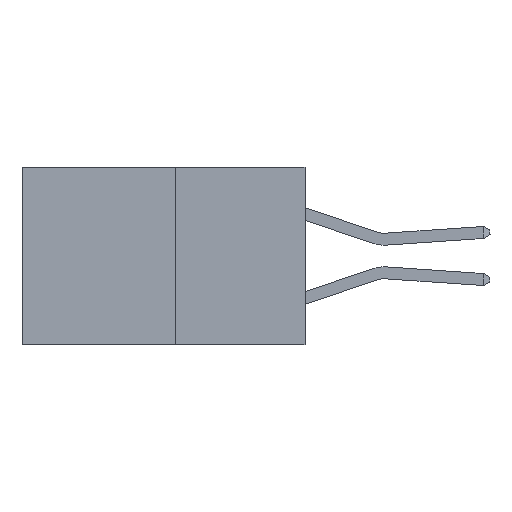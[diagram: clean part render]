
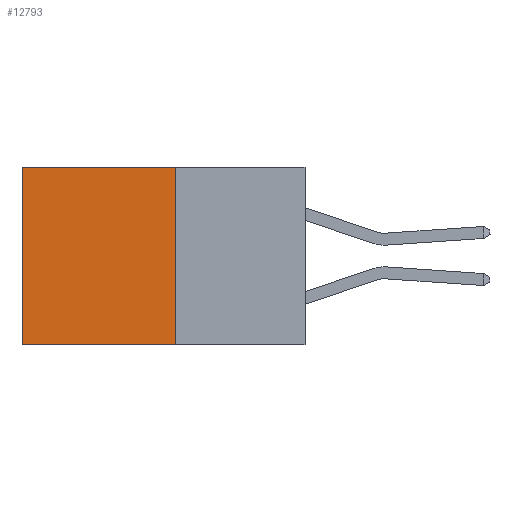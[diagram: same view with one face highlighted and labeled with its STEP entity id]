
A CAD part, left-side view. The second image highlights one B-rep face of the part: STEP entity #12793.
In plain terms, the highlighted planar face has unit normal (-1, 0, 0).
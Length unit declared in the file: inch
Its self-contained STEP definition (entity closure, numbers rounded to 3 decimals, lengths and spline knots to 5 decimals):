
#480 = PLANE ( 'NONE',  #8876 ) ;
#531 = VECTOR ( 'NONE', #13611, 39.37008 ) ;
#1140 = LINE ( 'NONE', #5750, #3578 ) ;
#1280 = EDGE_CURVE ( 'NONE', #2827, #8145, #3301, .T. ) ;
#2827 = VERTEX_POINT ( 'NONE', #12738 ) ;
#2942 = EDGE_LOOP ( 'NONE', ( #7919, #4447, #13223, #12456 ) ) ;
#3301 = LINE ( 'NONE', #7163, #531 ) ;
#3568 = VECTOR ( 'NONE', #4720, 39.37008 ) ;
#3578 = VECTOR ( 'NONE', #6773, 39.37008 ) ;
#3621 = CARTESIAN_POINT ( 'NONE',  ( 0.277, 0.27, -0.37 ) ) ;
#3948 = DIRECTION ( 'NONE',  ( 0., 1., 0. ) ) ;
#4089 = CARTESIAN_POINT ( 'NONE',  ( 0.277, 0.27, -0.37 ) ) ;
#4447 = ORIENTED_EDGE ( 'NONE', *, *, #6210, .F. ) ;
#4533 = CARTESIAN_POINT ( 'NONE',  ( 0.277, 0.27, 0. ) ) ;
#4691 = DIRECTION ( 'NONE',  ( 1., 0., 0. ) ) ;
#4720 = DIRECTION ( 'NONE',  ( 0., 1., 0. ) ) ;
#5750 = CARTESIAN_POINT ( 'NONE',  ( 0.277, 0.27, -0.37 ) ) ;
#6001 = EDGE_CURVE ( 'NONE', #9197, #6017, #1140, .T. ) ;
#6017 = VERTEX_POINT ( 'NONE', #7365 ) ;
#6210 = EDGE_CURVE ( 'NONE', #6017, #8145, #12204, .T. ) ;
#6541 = EDGE_CURVE ( 'NONE', #9197, #2827, #8198, .T. ) ;
#6773 = DIRECTION ( 'NONE',  ( 0., 0., -1. ) ) ;
#7163 = CARTESIAN_POINT ( 'NONE',  ( 0.277, 0.59, -0.37 ) ) ;
#7365 = CARTESIAN_POINT ( 'NONE',  ( 0.277, 0.27, -0.37 ) ) ;
#7919 = ORIENTED_EDGE ( 'NONE', *, *, #1280, .T. ) ;
#8145 = VERTEX_POINT ( 'NONE', #9403 ) ;
#8198 = LINE ( 'NONE', #4533, #3568 ) ;
#8876 = AXIS2_PLACEMENT_3D ( 'NONE', #3621, #4691, #12118 ) ;
#9197 = VERTEX_POINT ( 'NONE', #12126 ) ;
#9393 = VECTOR ( 'NONE', #3948, 39.37008 ) ;
#9403 = CARTESIAN_POINT ( 'NONE',  ( 0.277, 0.59, -0.37 ) ) ;
#9978 = FACE_OUTER_BOUND ( 'NONE', #2942, .T. ) ;
#12118 = DIRECTION ( 'NONE',  ( 0., 0., -1. ) ) ;
#12126 = CARTESIAN_POINT ( 'NONE',  ( 0.277, 0.27, 0. ) ) ;
#12204 = LINE ( 'NONE', #4089, #9393 ) ;
#12456 = ORIENTED_EDGE ( 'NONE', *, *, #6541, .T. ) ;
#12738 = CARTESIAN_POINT ( 'NONE',  ( 0.277, 0.59, 0. ) ) ;
#12793 = ADVANCED_FACE ( 'NONE', ( #9978 ), #480, .F. ) ;
#13223 = ORIENTED_EDGE ( 'NONE', *, *, #6001, .F. ) ;
#13611 = DIRECTION ( 'NONE',  ( 0., 0., -1. ) ) ;
